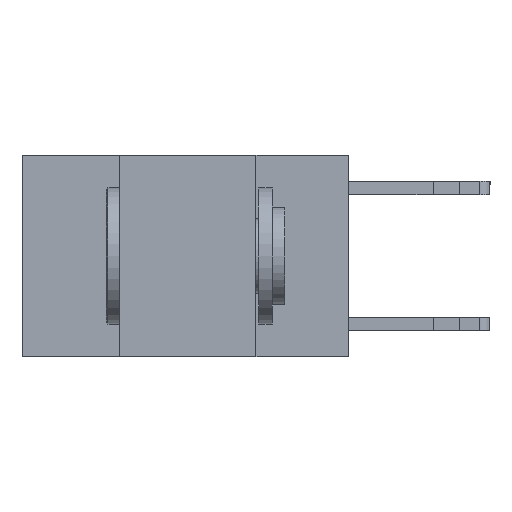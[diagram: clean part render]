
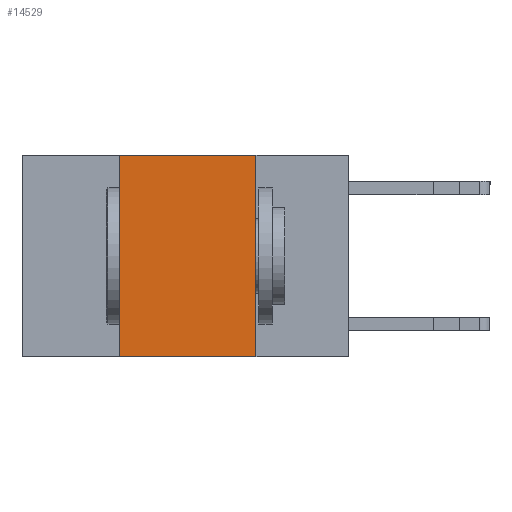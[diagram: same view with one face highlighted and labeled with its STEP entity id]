
A CAD part, left-side view. The second image highlights one B-rep face of the part: STEP entity #14529.
In plain terms, the highlighted planar face has unit normal (-1, 0, 0).
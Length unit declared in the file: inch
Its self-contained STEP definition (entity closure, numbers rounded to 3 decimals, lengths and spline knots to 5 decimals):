
#146 = DIRECTION ( 'NONE',  ( 0., 0., 1. ) ) ;
#631 = VECTOR ( 'NONE', #6448, 39.37008 ) ;
#1399 = VECTOR ( 'NONE', #146, 39.37008 ) ;
#1515 = CARTESIAN_POINT ( 'NONE',  ( 0., 0.17, 0. ) ) ;
#1553 = AXIS2_PLACEMENT_3D ( 'NONE', #1567, #17466, #13192 ) ;
#1567 = CARTESIAN_POINT ( 'NONE',  ( 0., 0.6, 0. ) ) ;
#1817 = ORIENTED_EDGE ( 'NONE', *, *, #17352, .T. ) ;
#2715 = EDGE_CURVE ( 'NONE', #18756, #12501, #12136, .T. ) ;
#4081 = CARTESIAN_POINT ( 'NONE',  ( 0., 0.6, -0.37 ) ) ;
#5018 = CARTESIAN_POINT ( 'NONE',  ( 0., 0.6, 0. ) ) ;
#5063 = CARTESIAN_POINT ( 'NONE',  ( 0., 0.17, 0. ) ) ;
#5571 = LINE ( 'NONE', #14436, #1399 ) ;
#6297 = CARTESIAN_POINT ( 'NONE',  ( 0., 0.42, 0. ) ) ;
#6448 = DIRECTION ( 'NONE',  ( 0., -1., 0. ) ) ;
#6707 = CARTESIAN_POINT ( 'NONE',  ( 0., 0.42, -0.37 ) ) ;
#6935 = DIRECTION ( 'NONE',  ( 0., -1., 0. ) ) ;
#7357 = EDGE_CURVE ( 'NONE', #17990, #18756, #8263, .T. ) ;
#8263 = LINE ( 'NONE', #5018, #631 ) ;
#9111 = VERTEX_POINT ( 'NONE', #6707 ) ;
#9825 = VECTOR ( 'NONE', #13653, 39.37008 ) ;
#11664 = PLANE ( 'NONE',  #1553 ) ;
#11810 = EDGE_LOOP ( 'NONE', ( #17708, #16082, #14371, #1817 ) ) ;
#12136 = LINE ( 'NONE', #5063, #9825 ) ;
#12501 = VERTEX_POINT ( 'NONE', #14249 ) ;
#12611 = EDGE_CURVE ( 'NONE', #9111, #17990, #5571, .T. ) ;
#12809 = VECTOR ( 'NONE', #6935, 39.37008 ) ;
#13192 = DIRECTION ( 'NONE',  ( 0., 0., -1. ) ) ;
#13653 = DIRECTION ( 'NONE',  ( 0., 0., -1. ) ) ;
#14249 = CARTESIAN_POINT ( 'NONE',  ( 0., 0.17, -0.37 ) ) ;
#14371 = ORIENTED_EDGE ( 'NONE', *, *, #12611, .F. ) ;
#14436 = CARTESIAN_POINT ( 'NONE',  ( 0., 0.42, 0. ) ) ;
#14529 = ADVANCED_FACE ( 'NONE', ( #17380 ), #11664, .F. ) ;
#15623 = LINE ( 'NONE', #4081, #12809 ) ;
#16082 = ORIENTED_EDGE ( 'NONE', *, *, #7357, .F. ) ;
#17352 = EDGE_CURVE ( 'NONE', #9111, #12501, #15623, .T. ) ;
#17380 = FACE_OUTER_BOUND ( 'NONE', #11810, .T. ) ;
#17466 = DIRECTION ( 'NONE',  ( 1., 0., 0. ) ) ;
#17708 = ORIENTED_EDGE ( 'NONE', *, *, #2715, .F. ) ;
#17990 = VERTEX_POINT ( 'NONE', #6297 ) ;
#18756 = VERTEX_POINT ( 'NONE', #1515 ) ;
